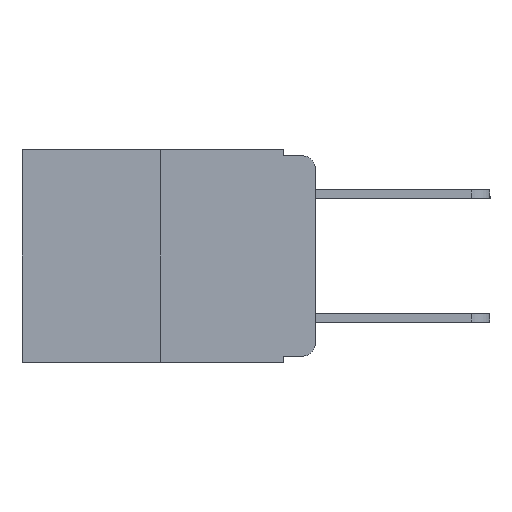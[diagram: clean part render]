
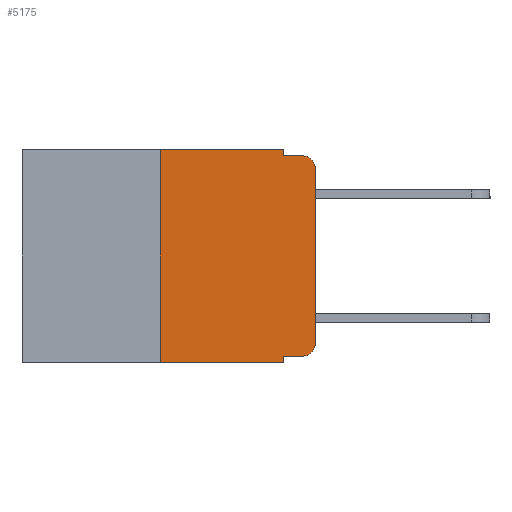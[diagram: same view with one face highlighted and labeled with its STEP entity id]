
A CAD part, left-side view. The second image highlights one B-rep face of the part: STEP entity #5175.
In plain terms, the highlighted planar face has unit normal (-1, 0, 0).
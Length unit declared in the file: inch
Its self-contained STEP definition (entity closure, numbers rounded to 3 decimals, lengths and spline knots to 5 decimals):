
#60 = DIRECTION ( 'NONE',  ( 0., -1., 0. ) ) ;
#71 = EDGE_CURVE ( 'NONE', #9682, #21754, #23854, .T. ) ;
#873 = DIRECTION ( 'NONE',  ( 0., 0., -1. ) ) ;
#909 = DIRECTION ( 'NONE',  ( -1., 0., 0. ) ) ;
#1421 = CARTESIAN_POINT ( 'NONE',  ( 0., 0.02, -0.03 ) ) ;
#2728 = PLANE ( 'NONE',  #3058 ) ;
#2811 = EDGE_CURVE ( 'NONE', #9758, #9682, #2910, .T. ) ;
#2910 = LINE ( 'NONE', #7732, #12722 ) ;
#3058 = AXIS2_PLACEMENT_3D ( 'NONE', #12526, #8667, #22095 ) ;
#3537 = LINE ( 'NONE', #21917, #12104 ) ;
#3776 = VECTOR ( 'NONE', #13582, 39.37008 ) ;
#4030 = CARTESIAN_POINT ( 'NONE',  ( 0., 0.051, -0.01 ) ) ;
#4516 = DIRECTION ( 'NONE',  ( 0., -1., 0. ) ) ;
#4766 = ORIENTED_EDGE ( 'NONE', *, *, #22388, .T. ) ;
#4806 = DIRECTION ( 'NONE',  ( -1., 0., 0. ) ) ;
#5028 = LINE ( 'NONE', #6820, #10872 ) ;
#5175 = ADVANCED_FACE ( 'NONE', ( #15712 ), #2728, .F. ) ;
#5301 = CARTESIAN_POINT ( 'NONE',  ( 0., 0.051, 0. ) ) ;
#5315 = ORIENTED_EDGE ( 'NONE', *, *, #71, .T. ) ;
#5641 = LINE ( 'NONE', #5301, #24831 ) ;
#5657 = VERTEX_POINT ( 'NONE', #21575 ) ;
#5762 = EDGE_CURVE ( 'NONE', #18409, #5657, #3537, .T. ) ;
#5903 = VECTOR ( 'NONE', #19510, 39.37008 ) ;
#6308 = EDGE_CURVE ( 'NONE', #24985, #13656, #5028, .T. ) ;
#6496 = ORIENTED_EDGE ( 'NONE', *, *, #20229, .F. ) ;
#6551 = ORIENTED_EDGE ( 'NONE', *, *, #17630, .F. ) ;
#6820 = CARTESIAN_POINT ( 'NONE',  ( 0., 0.473, 0. ) ) ;
#6823 = CARTESIAN_POINT ( 'NONE',  ( 0., 0.051, 0. ) ) ;
#7153 = LINE ( 'NONE', #4030, #16868 ) ;
#7732 = CARTESIAN_POINT ( 'NONE',  ( 0., 0., 0. ) ) ;
#8552 = EDGE_CURVE ( 'NONE', #20535, #16823, #24799, .T. ) ;
#8667 = DIRECTION ( 'NONE',  ( 1., 0., 0. ) ) ;
#8942 = DIRECTION ( 'NONE',  ( 0., 0., -1. ) ) ;
#9662 = CARTESIAN_POINT ( 'NONE',  ( 0., 0.051, -0.333 ) ) ;
#9682 = VERTEX_POINT ( 'NONE', #16704 ) ;
#9758 = VERTEX_POINT ( 'NONE', #20869 ) ;
#9835 = LINE ( 'NONE', #16719, #24474 ) ;
#10386 = CARTESIAN_POINT ( 'NONE',  ( 0., 0.25, 0. ) ) ;
#10605 = ORIENTED_EDGE ( 'NONE', *, *, #6308, .F. ) ;
#10625 = CARTESIAN_POINT ( 'NONE',  ( 0., 0.25, -0.343 ) ) ;
#10634 = CARTESIAN_POINT ( 'NONE',  ( 0., 0.02, -0.01 ) ) ;
#10872 = VECTOR ( 'NONE', #18436, 39.37008 ) ;
#10983 = CARTESIAN_POINT ( 'NONE',  ( 0., 0.051, -0.333 ) ) ;
#11144 = LINE ( 'NONE', #13709, #5903 ) ;
#11403 = ORIENTED_EDGE ( 'NONE', *, *, #15061, .F. ) ;
#11437 = VERTEX_POINT ( 'NONE', #18004 ) ;
#11639 = AXIS2_PLACEMENT_3D ( 'NONE', #1421, #909, #873 ) ;
#12104 = VECTOR ( 'NONE', #4516, 39.37008 ) ;
#12526 = CARTESIAN_POINT ( 'NONE',  ( 0., 0.473, 0. ) ) ;
#12596 = CIRCLE ( 'NONE', #16702, 0.02 ) ;
#12722 = VECTOR ( 'NONE', #19473, 39.37008 ) ;
#13410 = ORIENTED_EDGE ( 'NONE', *, *, #5762, .T. ) ;
#13582 = DIRECTION ( 'NONE',  ( 0., -1., 0. ) ) ;
#13656 = VERTEX_POINT ( 'NONE', #6823 ) ;
#13709 = CARTESIAN_POINT ( 'NONE',  ( 0., 0.25, 0. ) ) ;
#13776 = EDGE_CURVE ( 'NONE', #20535, #5657, #5641, .T. ) ;
#15061 = EDGE_CURVE ( 'NONE', #18409, #24985, #11144, .T. ) ;
#15161 = EDGE_LOOP ( 'NONE', ( #24963, #5315, #6496, #6551, #10605, #11403, #13410, #17334, #23224, #4766 ) ) ;
#15712 = FACE_OUTER_BOUND ( 'NONE', #15161, .T. ) ;
#15801 = CARTESIAN_POINT ( 'NONE',  ( 0., 0.02, -0.333 ) ) ;
#16413 = CARTESIAN_POINT ( 'NONE',  ( 0., 0.02, -0.313 ) ) ;
#16702 = AXIS2_PLACEMENT_3D ( 'NONE', #16413, #4806, #18360 ) ;
#16704 = CARTESIAN_POINT ( 'NONE',  ( 0., 0., -0.03 ) ) ;
#16719 = CARTESIAN_POINT ( 'NONE',  ( 0., 0.051, 0. ) ) ;
#16823 = VERTEX_POINT ( 'NONE', #15801 ) ;
#16868 = VECTOR ( 'NONE', #60, 39.37008 ) ;
#16930 = DIRECTION ( 'NONE',  ( 0., 0., -1. ) ) ;
#17334 = ORIENTED_EDGE ( 'NONE', *, *, #13776, .F. ) ;
#17630 = EDGE_CURVE ( 'NONE', #13656, #11437, #9835, .T. ) ;
#18004 = CARTESIAN_POINT ( 'NONE',  ( 0., 0.051, -0.01 ) ) ;
#18360 = DIRECTION ( 'NONE',  ( 0., 0., -1. ) ) ;
#18409 = VERTEX_POINT ( 'NONE', #10625 ) ;
#18436 = DIRECTION ( 'NONE',  ( 0., -1., 0. ) ) ;
#19473 = DIRECTION ( 'NONE',  ( 0., 0., 1. ) ) ;
#19510 = DIRECTION ( 'NONE',  ( 0., 0., 1. ) ) ;
#20229 = EDGE_CURVE ( 'NONE', #11437, #21754, #7153, .T. ) ;
#20535 = VERTEX_POINT ( 'NONE', #10983 ) ;
#20869 = CARTESIAN_POINT ( 'NONE',  ( 0., 0., -0.313 ) ) ;
#21575 = CARTESIAN_POINT ( 'NONE',  ( 0., 0.051, -0.343 ) ) ;
#21754 = VERTEX_POINT ( 'NONE', #10634 ) ;
#21917 = CARTESIAN_POINT ( 'NONE',  ( 0., 0.473, -0.343 ) ) ;
#22095 = DIRECTION ( 'NONE',  ( 0., 0., -1. ) ) ;
#22388 = EDGE_CURVE ( 'NONE', #16823, #9758, #12596, .T. ) ;
#23224 = ORIENTED_EDGE ( 'NONE', *, *, #8552, .T. ) ;
#23854 = CIRCLE ( 'NONE', #11639, 0.02 ) ;
#24474 = VECTOR ( 'NONE', #8942, 39.37008 ) ;
#24799 = LINE ( 'NONE', #9662, #3776 ) ;
#24831 = VECTOR ( 'NONE', #16930, 39.37008 ) ;
#24963 = ORIENTED_EDGE ( 'NONE', *, *, #2811, .T. ) ;
#24985 = VERTEX_POINT ( 'NONE', #10386 ) ;
